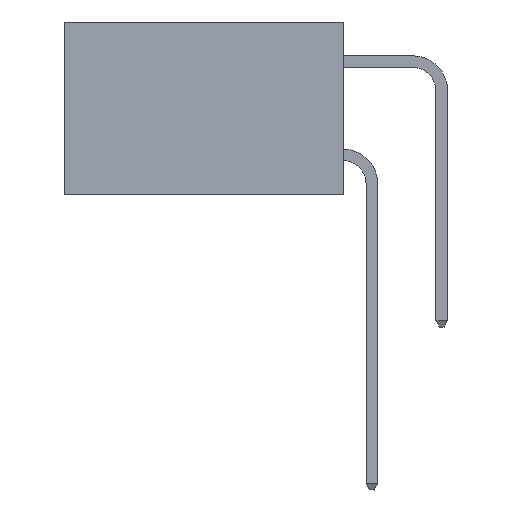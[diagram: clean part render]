
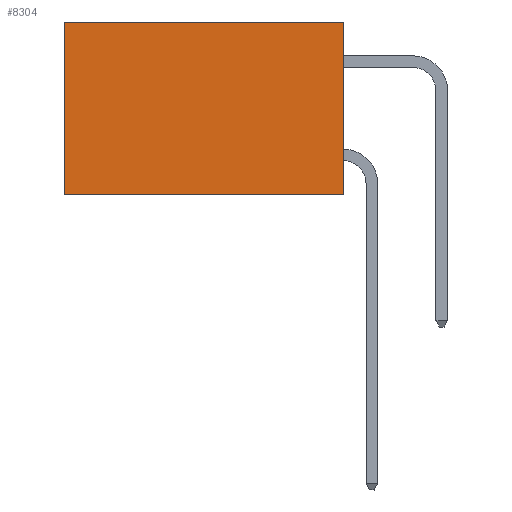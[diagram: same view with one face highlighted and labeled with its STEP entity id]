
A CAD part, left-side view. The second image highlights one B-rep face of the part: STEP entity #8304.
In plain terms, the highlighted planar face has unit normal (-1, 0, 0).
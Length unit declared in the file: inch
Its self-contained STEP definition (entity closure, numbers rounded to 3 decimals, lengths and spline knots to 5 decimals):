
#775 = VERTEX_POINT ( 'NONE', #9295 ) ;
#977 = DIRECTION ( 'NONE',  ( 0., 0., -1. ) ) ;
#1578 = ORIENTED_EDGE ( 'NONE', *, *, #12435, .F. ) ;
#1738 = CARTESIAN_POINT ( 'NONE',  ( 0.298, 0., 0. ) ) ;
#2642 = ORIENTED_EDGE ( 'NONE', *, *, #14627, .T. ) ;
#2909 = DIRECTION ( 'NONE',  ( 0., 0., -1. ) ) ;
#3453 = DIRECTION ( 'NONE',  ( 0., 1., 0. ) ) ;
#4489 = CARTESIAN_POINT ( 'NONE',  ( 0.298, 0.6, -0.37 ) ) ;
#4490 = CARTESIAN_POINT ( 'NONE',  ( 0.298, 0., 0. ) ) ;
#4824 = EDGE_LOOP ( 'NONE', ( #10237, #7385, #1578, #2642 ) ) ;
#6039 = CARTESIAN_POINT ( 'NONE',  ( 0.298, 0.6, 0. ) ) ;
#6080 = EDGE_CURVE ( 'NONE', #14417, #13167, #8555, .T. ) ;
#6446 = DIRECTION ( 'NONE',  ( 0., 1., 0. ) ) ;
#6716 = VECTOR ( 'NONE', #6446, 39.37008 ) ;
#7180 = VECTOR ( 'NONE', #7961, 39.37008 ) ;
#7325 = CARTESIAN_POINT ( 'NONE',  ( 0.298, 0., -0.37 ) ) ;
#7385 = ORIENTED_EDGE ( 'NONE', *, *, #16437, .F. ) ;
#7961 = DIRECTION ( 'NONE',  ( 0., 0., -1. ) ) ;
#8219 = VERTEX_POINT ( 'NONE', #9431 ) ;
#8286 = PLANE ( 'NONE',  #12735 ) ;
#8304 = ADVANCED_FACE ( 'NONE', ( #15961 ), #8286, .F. ) ;
#8555 = LINE ( 'NONE', #15704, #7180 ) ;
#9295 = CARTESIAN_POINT ( 'NONE',  ( 0.298, 0., 0. ) ) ;
#9431 = CARTESIAN_POINT ( 'NONE',  ( 0.298, 0., -0.37 ) ) ;
#10237 = ORIENTED_EDGE ( 'NONE', *, *, #6080, .T. ) ;
#11767 = VECTOR ( 'NONE', #2909, 39.37008 ) ;
#12435 = EDGE_CURVE ( 'NONE', #775, #8219, #15205, .T. ) ;
#12729 = CARTESIAN_POINT ( 'NONE',  ( 0.298, 0., 0. ) ) ;
#12735 = AXIS2_PLACEMENT_3D ( 'NONE', #4490, #14725, #977 ) ;
#13167 = VERTEX_POINT ( 'NONE', #4489 ) ;
#13655 = LINE ( 'NONE', #7325, #15492 ) ;
#14417 = VERTEX_POINT ( 'NONE', #6039 ) ;
#14627 = EDGE_CURVE ( 'NONE', #775, #14417, #14745, .T. ) ;
#14725 = DIRECTION ( 'NONE',  ( 1., 0., 0. ) ) ;
#14745 = LINE ( 'NONE', #12729, #6716 ) ;
#15205 = LINE ( 'NONE', #1738, #11767 ) ;
#15492 = VECTOR ( 'NONE', #3453, 39.37008 ) ;
#15704 = CARTESIAN_POINT ( 'NONE',  ( 0.298, 0.6, 0. ) ) ;
#15961 = FACE_OUTER_BOUND ( 'NONE', #4824, .T. ) ;
#16437 = EDGE_CURVE ( 'NONE', #8219, #13167, #13655, .T. ) ;
